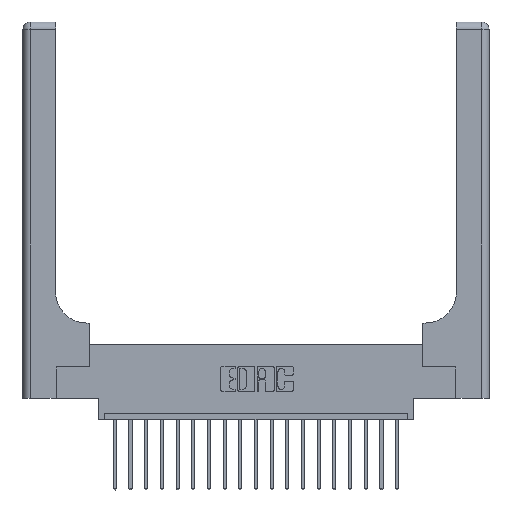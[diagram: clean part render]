
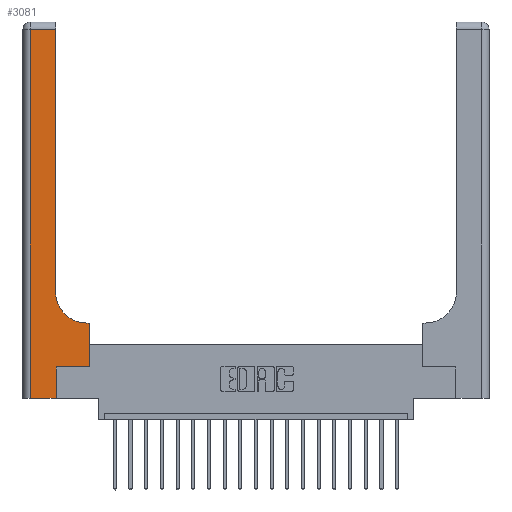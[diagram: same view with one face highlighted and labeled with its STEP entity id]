
A CAD part, top view. The second image highlights one B-rep face of the part: STEP entity #3081.
In plain terms, the highlighted planar face has unit normal (0, 0, 1).
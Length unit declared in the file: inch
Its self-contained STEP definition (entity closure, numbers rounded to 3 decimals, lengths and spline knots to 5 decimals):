
#637 = ORIENTED_EDGE ( 'NONE', *, *, #2387, .T. ) ;
#1211 = CARTESIAN_POINT ( 'NONE',  ( 0., 2.94, 0.37 ) ) ;
#1402 = DIRECTION ( 'NONE',  ( 0., 1., 0. ) ) ;
#1983 = CARTESIAN_POINT ( 'NONE',  ( 0.265, 0.25, 0.37 ) ) ;
#2074 = LINE ( 'NONE', #17936, #12830 ) ;
#2387 = EDGE_CURVE ( 'NONE', #2398, #7684, #19199, .T. ) ;
#2390 = AXIS2_PLACEMENT_3D ( 'NONE', #3000, #7641, #7717 ) ;
#2398 = VERTEX_POINT ( 'NONE', #11862 ) ;
#2496 = EDGE_CURVE ( 'NONE', #8539, #12777, #3316, .T. ) ;
#2823 = CARTESIAN_POINT ( 'NONE',  ( 0.528, 0.6, 0.37 ) ) ;
#3000 = CARTESIAN_POINT ( 'NONE',  ( 0.51, 0.85, 0.37 ) ) ;
#3081 = ADVANCED_FACE ( 'NONE', ( #10912 ), #18035, .F. ) ;
#3198 = CIRCLE ( 'NONE', #2390, 0.25 ) ;
#3316 = LINE ( 'NONE', #5166, #10164 ) ;
#3408 = VECTOR ( 'NONE', #4418, 39.37008 ) ;
#3517 = VECTOR ( 'NONE', #7583, 39.37008 ) ;
#4251 = EDGE_CURVE ( 'NONE', #15206, #2398, #16701, .T. ) ;
#4418 = DIRECTION ( 'NONE',  ( -1., 0., 0. ) ) ;
#4598 = CARTESIAN_POINT ( 'NONE',  ( 0.265, 0., 0.37 ) ) ;
#5008 = VECTOR ( 'NONE', #6738, 39.37008 ) ;
#5022 = ORIENTED_EDGE ( 'NONE', *, *, #13728, .T. ) ;
#5166 = CARTESIAN_POINT ( 'NONE',  ( 0.26, 0.6, 0.37 ) ) ;
#5627 = DIRECTION ( 'NONE',  ( 0., 1., 0. ) ) ;
#5952 = CARTESIAN_POINT ( 'NONE',  ( 0.26, 0.85, 0.37 ) ) ;
#6738 = DIRECTION ( 'NONE',  ( 1., 0., 0. ) ) ;
#7054 = LINE ( 'NONE', #1211, #3408 ) ;
#7440 = CARTESIAN_POINT ( 'NONE',  ( 0.26, 2.94, 0.37 ) ) ;
#7441 = CARTESIAN_POINT ( 'NONE',  ( 0.06, 3., 0.37 ) ) ;
#7583 = DIRECTION ( 'NONE',  ( 0., -1., 0. ) ) ;
#7641 = DIRECTION ( 'NONE',  ( 0., 0., -1. ) ) ;
#7684 = VERTEX_POINT ( 'NONE', #7918 ) ;
#7717 = DIRECTION ( 'NONE',  ( 1., 0., 0. ) ) ;
#7867 = EDGE_CURVE ( 'NONE', #8173, #9948, #14103, .T. ) ;
#7918 = CARTESIAN_POINT ( 'NONE',  ( 0.265, 0., 0.37 ) ) ;
#8173 = VERTEX_POINT ( 'NONE', #15387 ) ;
#8539 = VERTEX_POINT ( 'NONE', #2823 ) ;
#8757 = DIRECTION ( 'NONE',  ( -1., 0., 0. ) ) ;
#9118 = ORIENTED_EDGE ( 'NONE', *, *, #7867, .T. ) ;
#9492 = ORIENTED_EDGE ( 'NONE', *, *, #19866, .T. ) ;
#9836 = CARTESIAN_POINT ( 'NONE',  ( 0.51, 0.6, 0.37 ) ) ;
#9892 = DIRECTION ( 'NONE',  ( 0., 1., 0. ) ) ;
#9948 = VERTEX_POINT ( 'NONE', #10725 ) ;
#10164 = VECTOR ( 'NONE', #14643, 39.37008 ) ;
#10423 = VECTOR ( 'NONE', #13409, 39.37008 ) ;
#10580 = ORIENTED_EDGE ( 'NONE', *, *, #4251, .T. ) ;
#10725 = CARTESIAN_POINT ( 'NONE',  ( 0.528, 0.25, 0.37 ) ) ;
#10912 = FACE_OUTER_BOUND ( 'NONE', #13185, .T. ) ;
#11299 = ORIENTED_EDGE ( 'NONE', *, *, #12291, .T. ) ;
#11793 = CARTESIAN_POINT ( 'NONE',  ( 0., 0., 0.37 ) ) ;
#11862 = CARTESIAN_POINT ( 'NONE',  ( 0.06, 0., 0.37 ) ) ;
#12000 = AXIS2_PLACEMENT_3D ( 'NONE', #16678, #12010, #8757 ) ;
#12010 = DIRECTION ( 'NONE',  ( 0., 0., -1. ) ) ;
#12072 = VERTEX_POINT ( 'NONE', #7440 ) ;
#12291 = EDGE_CURVE ( 'NONE', #12072, #15206, #7054, .T. ) ;
#12443 = ORIENTED_EDGE ( 'NONE', *, *, #2496, .T. ) ;
#12777 = VERTEX_POINT ( 'NONE', #9836 ) ;
#12830 = VECTOR ( 'NONE', #5627, 39.37008 ) ;
#13185 = EDGE_LOOP ( 'NONE', ( #9492, #11299, #10580, #637, #5022, #9118, #17271, #12443, #14549 ) ) ;
#13409 = DIRECTION ( 'NONE',  ( 1., 0., 0. ) ) ;
#13554 = CARTESIAN_POINT ( 'NONE',  ( 0.06, 2.94, 0.37 ) ) ;
#13728 = EDGE_CURVE ( 'NONE', #7684, #8173, #18957, .T. ) ;
#14103 = LINE ( 'NONE', #1983, #5008 ) ;
#14483 = LINE ( 'NONE', #18823, #16620 ) ;
#14549 = ORIENTED_EDGE ( 'NONE', *, *, #15875, .T. ) ;
#14643 = DIRECTION ( 'NONE',  ( -1., 0., 0. ) ) ;
#15206 = VERTEX_POINT ( 'NONE', #13554 ) ;
#15387 = CARTESIAN_POINT ( 'NONE',  ( 0.265, 0.25, 0.37 ) ) ;
#15599 = VECTOR ( 'NONE', #1402, 39.37008 ) ;
#15875 = EDGE_CURVE ( 'NONE', #12777, #18078, #3198, .T. ) ;
#16011 = EDGE_CURVE ( 'NONE', #9948, #8539, #14483, .T. ) ;
#16620 = VECTOR ( 'NONE', #9892, 39.37008 ) ;
#16678 = CARTESIAN_POINT ( 'NONE',  ( 0., 3., 0.37 ) ) ;
#16701 = LINE ( 'NONE', #7441, #3517 ) ;
#17271 = ORIENTED_EDGE ( 'NONE', *, *, #16011, .T. ) ;
#17936 = CARTESIAN_POINT ( 'NONE',  ( 0.26, 3., 0.37 ) ) ;
#18035 = PLANE ( 'NONE',  #12000 ) ;
#18078 = VERTEX_POINT ( 'NONE', #5952 ) ;
#18823 = CARTESIAN_POINT ( 'NONE',  ( 0.528, 0.25, 0.37 ) ) ;
#18957 = LINE ( 'NONE', #4598, #15599 ) ;
#19199 = LINE ( 'NONE', #11793, #10423 ) ;
#19866 = EDGE_CURVE ( 'NONE', #18078, #12072, #2074, .T. ) ;
